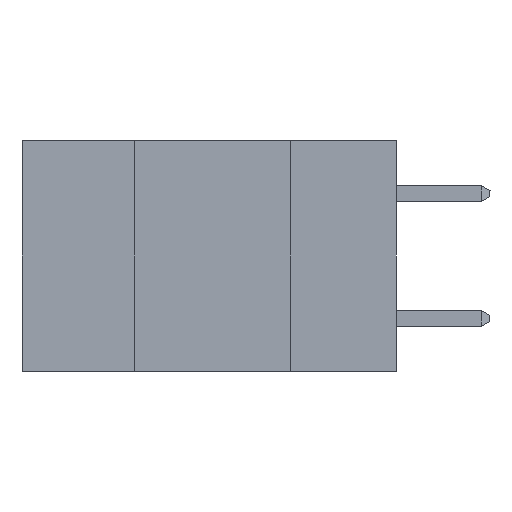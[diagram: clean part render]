
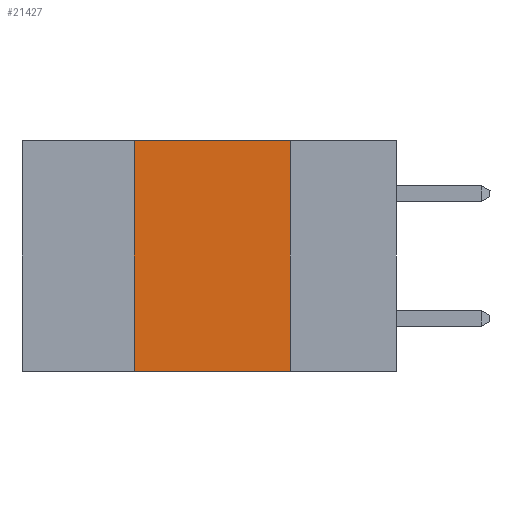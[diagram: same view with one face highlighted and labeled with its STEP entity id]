
A CAD part, left-side view. The second image highlights one B-rep face of the part: STEP entity #21427.
In plain terms, the highlighted planar face has unit normal (-1, 0, 0).
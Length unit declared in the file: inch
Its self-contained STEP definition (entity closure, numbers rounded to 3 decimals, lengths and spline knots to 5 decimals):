
#1289 = EDGE_CURVE ( 'NONE', #19630, #23330, #14241, .T. ) ;
#1470 = CARTESIAN_POINT ( 'NONE',  ( 0., 0.6, 0. ) ) ;
#1985 = DIRECTION ( 'NONE',  ( 0., 0., 1. ) ) ;
#2308 = LINE ( 'NONE', #13065, #11704 ) ;
#2822 = ORIENTED_EDGE ( 'NONE', *, *, #6076, .F. ) ;
#2967 = DIRECTION ( 'NONE',  ( 1., 0., 0. ) ) ;
#3559 = LINE ( 'NONE', #1470, #19130 ) ;
#4242 = VECTOR ( 'NONE', #1985, 39.37008 ) ;
#4719 = EDGE_CURVE ( 'NONE', #23330, #12572, #3559, .T. ) ;
#5266 = CARTESIAN_POINT ( 'NONE',  ( 0., 0.17, 0. ) ) ;
#6076 = EDGE_CURVE ( 'NONE', #12572, #23268, #2308, .T. ) ;
#7429 = CARTESIAN_POINT ( 'NONE',  ( 0., 0.42, 0. ) ) ;
#7509 = AXIS2_PLACEMENT_3D ( 'NONE', #21648, #2967, #16117 ) ;
#8878 = DIRECTION ( 'NONE',  ( 0., -1., 0. ) ) ;
#9075 = CARTESIAN_POINT ( 'NONE',  ( 0., 0.17, -0.37 ) ) ;
#9116 = EDGE_LOOP ( 'NONE', ( #2822, #11326, #22778, #23082 ) ) ;
#11081 = CARTESIAN_POINT ( 'NONE',  ( 0., 0.42, -0.37 ) ) ;
#11118 = CARTESIAN_POINT ( 'NONE',  ( 0., 0.42, 0. ) ) ;
#11326 = ORIENTED_EDGE ( 'NONE', *, *, #4719, .F. ) ;
#11704 = VECTOR ( 'NONE', #14973, 39.37008 ) ;
#12231 = CARTESIAN_POINT ( 'NONE',  ( 0., 0.6, -0.37 ) ) ;
#12302 = PLANE ( 'NONE',  #7509 ) ;
#12572 = VERTEX_POINT ( 'NONE', #5266 ) ;
#13065 = CARTESIAN_POINT ( 'NONE',  ( 0., 0.17, 0. ) ) ;
#14241 = LINE ( 'NONE', #7429, #4242 ) ;
#14613 = DIRECTION ( 'NONE',  ( 0., -1., 0. ) ) ;
#14973 = DIRECTION ( 'NONE',  ( 0., 0., -1. ) ) ;
#15171 = VECTOR ( 'NONE', #8878, 39.37008 ) ;
#15240 = EDGE_CURVE ( 'NONE', #19630, #23268, #20171, .T. ) ;
#16117 = DIRECTION ( 'NONE',  ( 0., 0., -1. ) ) ;
#19130 = VECTOR ( 'NONE', #14613, 39.37008 ) ;
#19173 = FACE_OUTER_BOUND ( 'NONE', #9116, .T. ) ;
#19630 = VERTEX_POINT ( 'NONE', #11081 ) ;
#20171 = LINE ( 'NONE', #12231, #15171 ) ;
#21427 = ADVANCED_FACE ( 'NONE', ( #19173 ), #12302, .F. ) ;
#21648 = CARTESIAN_POINT ( 'NONE',  ( 0., 0.6, 0. ) ) ;
#22778 = ORIENTED_EDGE ( 'NONE', *, *, #1289, .F. ) ;
#23082 = ORIENTED_EDGE ( 'NONE', *, *, #15240, .T. ) ;
#23268 = VERTEX_POINT ( 'NONE', #9075 ) ;
#23330 = VERTEX_POINT ( 'NONE', #11118 ) ;
